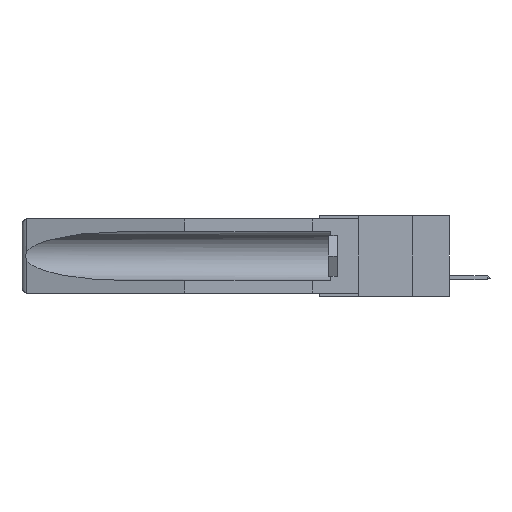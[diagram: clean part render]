
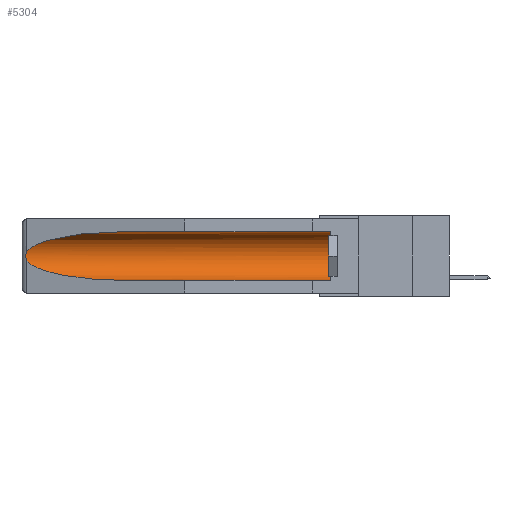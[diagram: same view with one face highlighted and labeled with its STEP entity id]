
A CAD part, left-side view. The second image highlights one B-rep face of the part: STEP entity #5304.
In plain terms, the highlighted cylindrical face has radius 2.857 mm (diameter 5.715 mm), a partial arc.
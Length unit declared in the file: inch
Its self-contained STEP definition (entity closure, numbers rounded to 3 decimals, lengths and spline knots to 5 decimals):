
#21 = VECTOR ( 'NONE', #1537, 39.37008 ) ;
#723 = CARTESIAN_POINT ( 'NONE',  ( 0.155, 1.07973, -0.284 ) ) ;
#964 = ORIENTED_EDGE ( 'NONE', *, *, #3125, .T. ) ;
#1537 = DIRECTION ( 'NONE',  ( 0., 1., 0. ) ) ;
#2819 = CARTESIAN_POINT ( 'NONE',  ( 0.26655, 1.53094, -0.18657 ) ) ;
#2965 = ORIENTED_EDGE ( 'NONE', *, *, #8725, .T. ) ;
#3125 = EDGE_CURVE ( 'NONE', #13203, #8011, #6823, .T. ) ;
#3153 = CARTESIAN_POINT ( 'NONE',  ( 0.26537, 1.52718, -0.14972 ) ) ;
#3886 = CARTESIAN_POINT ( 'NONE',  ( 0.155, 1.07973, -0.059 ) ) ;
#4081 = LINE ( 'NONE', #13423, #14589 ) ;
#4267 = EDGE_CURVE ( 'NONE', #8011, #5471, #12851, .T. ) ;
#4612 = CARTESIAN_POINT ( 'NONE',  ( 0.26537, 1.52718, -0.19328 ) ) ;
#5048 = CARTESIAN_POINT ( 'NONE',  ( 0.155, 0.126, -0.284 ) ) ;
#5304 = ADVANCED_FACE ( 'NONE', ( #12239 ), #5321, .F. ) ;
#5321 = CYLINDRICAL_SURFACE ( 'NONE', #9983, 0.1125 ) ;
#5471 = VERTEX_POINT ( 'NONE', #723 ) ;
#5567 = CARTESIAN_POINT ( 'NONE',  ( 0.26537, 1.52718, -0.19328 ) ) ;
#5690 = CARTESIAN_POINT ( 'NONE',  ( 0.25451, 1.48313, -0.24835 ) ) ;
#5893 = DIRECTION ( 'NONE',  ( 0., -1., 0. ) ) ;
#6440 = DIRECTION ( 'NONE',  ( 0., 0., 1. ) ) ;
#6823 = B_SPLINE_CURVE_WITH_KNOTS ( 'NONE', 3,
 ( #12336, #14927, #7749, #14761, #8793, #10011, #11098, #2819, #13494, #13862 ),
 .UNSPECIFIED., .F., .F.,
 ( 4, 2, 2, 2, 4 ),
 ( 0., 0.00029, 0.00058, 0.00087, 0.00117 ),
 .UNSPECIFIED. ) ;
#6938 = ORIENTED_EDGE ( 'NONE', *, *, #13986, .T. ) ;
#6969 = EDGE_CURVE ( 'NONE', #7838, #5471, #11456, .T. ) ;
#7749 = CARTESIAN_POINT ( 'NONE',  ( 0.26654, 1.53092, -0.15636 ) ) ;
#7838 = VERTEX_POINT ( 'NONE', #5048 ) ;
#8011 = VERTEX_POINT ( 'NONE', #5567 ) ;
#8114 = VERTEX_POINT ( 'NONE', #10455 ) ;
#8190 = CARTESIAN_POINT ( 'NONE',  ( 0.21114, 1.30732, -0.284 ) ) ;
#8287 = DIRECTION ( 'NONE',  ( 0., 0., 1. ) ) ;
#8725 = EDGE_CURVE ( 'NONE', #8114, #12356, #4081, .T. ) ;
#8793 = CARTESIAN_POINT ( 'NONE',  ( 0.2675, 1.53308, -0.16763 ) ) ;
#9328 = CARTESIAN_POINT ( 'NONE',  ( 0.155, 1.07973, -0.059 ) ) ;
#9362 = ORIENTED_EDGE ( 'NONE', *, *, #12183, .T. ) ;
#9647 = EDGE_LOOP ( 'NONE', ( #9362, #964, #13258, #12337, #6938, #2965 ) ) ;
#9830 = CARTESIAN_POINT ( 'NONE',  ( 0.21114, 1.30732, -0.059 ) ) ;
#9983 = AXIS2_PLACEMENT_3D ( 'NONE', #12542, #11248, #6440 ) ;
#10011 = CARTESIAN_POINT ( 'NONE',  ( 0.2675, 1.53308, -0.17534 ) ) ;
#10014 = CIRCLE ( 'NONE', #12143, 0.1125 ) ;
#10455 = CARTESIAN_POINT ( 'NONE',  ( 0.155, 0.126, -0.059 ) ) ;
#10602 = CARTESIAN_POINT ( 'NONE',  ( 0.155, 1.07973, -0.284 ) ) ;
#11098 = CARTESIAN_POINT ( 'NONE',  ( 0.2673, 1.53269, -0.17917 ) ) ;
#11210 = CARTESIAN_POINT ( 'NONE',  ( 0.25451, 1.48313, -0.09465 ) ) ;
#11248 = DIRECTION ( 'NONE',  ( 0., 1., 0. ) ) ;
#11324 = CARTESIAN_POINT ( 'NONE',  ( 0.155, -0.30754, -0.284 ) ) ;
#11456 = LINE ( 'NONE', #11324, #21 ) ;
#12143 = AXIS2_PLACEMENT_3D ( 'NONE', #15438, #5893, #8287 ) ;
#12182 = DIRECTION ( 'NONE',  ( 0., 1., 0. ) ) ;
#12183 = EDGE_CURVE ( 'NONE', #12356, #13203, #13329, .T. ) ;
#12239 = FACE_OUTER_BOUND ( 'NONE', #9647, .T. ) ;
#12257 = CARTESIAN_POINT ( 'NONE',  ( 0.26537, 1.52718, -0.14972 ) ) ;
#12336 = CARTESIAN_POINT ( 'NONE',  ( 0.26537, 1.52718, -0.14972 ) ) ;
#12337 = ORIENTED_EDGE ( 'NONE', *, *, #6969, .F. ) ;
#12356 = VERTEX_POINT ( 'NONE', #9328 ) ;
#12542 = CARTESIAN_POINT ( 'NONE',  ( 0.155, -0.30754, -0.1715 ) ) ;
#12851 =( BOUNDED_CURVE ( )  B_SPLINE_CURVE ( 3, ( #4612, #5690, #8190, #10602 ),
 .UNSPECIFIED., .F., .F. ) 
 B_SPLINE_CURVE_WITH_KNOTS ( ( 4, 4 ),
 ( 0.1948, 1.5708 ),
 .UNSPECIFIED. ) 
 CURVE ( )  GEOMETRIC_REPRESENTATION_ITEM ( )  RATIONAL_B_SPLINE_CURVE ( ( 1., 0.848, 0.848, 1. ) ) 
 REPRESENTATION_ITEM ( '' )  );
#13203 = VERTEX_POINT ( 'NONE', #3153 ) ;
#13258 = ORIENTED_EDGE ( 'NONE', *, *, #4267, .T. ) ;
#13329 =( BOUNDED_CURVE ( )  B_SPLINE_CURVE ( 3, ( #3886, #9830, #11210, #12257 ),
 .UNSPECIFIED., .F., .F. ) 
 B_SPLINE_CURVE_WITH_KNOTS ( ( 4, 4 ),
 ( 4.71239, 6.08839 ),
 .UNSPECIFIED. ) 
 CURVE ( )  GEOMETRIC_REPRESENTATION_ITEM ( )  RATIONAL_B_SPLINE_CURVE ( ( 1., 0.848, 0.848, 1. ) ) 
 REPRESENTATION_ITEM ( '' )  );
#13423 = CARTESIAN_POINT ( 'NONE',  ( 0.155, -0.30754, -0.059 ) ) ;
#13494 = CARTESIAN_POINT ( 'NONE',  ( 0.26597, 1.5296, -0.19026 ) ) ;
#13862 = CARTESIAN_POINT ( 'NONE',  ( 0.26537, 1.52718, -0.19328 ) ) ;
#13986 = EDGE_CURVE ( 'NONE', #7838, #8114, #10014, .T. ) ;
#14589 = VECTOR ( 'NONE', #12182, 39.37008 ) ;
#14761 = CARTESIAN_POINT ( 'NONE',  ( 0.2673, 1.5327, -0.16383 ) ) ;
#14927 = CARTESIAN_POINT ( 'NONE',  ( 0.26597, 1.52961, -0.15275 ) ) ;
#15438 = CARTESIAN_POINT ( 'NONE',  ( 0.155, 0.126, -0.1715 ) ) ;
